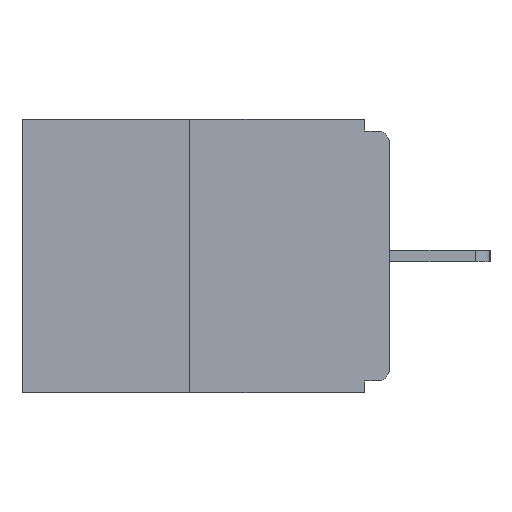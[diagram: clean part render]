
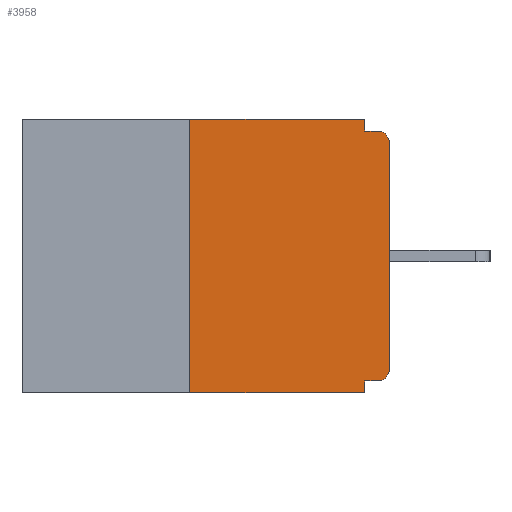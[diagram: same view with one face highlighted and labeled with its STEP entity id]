
A CAD part, left-side view. The second image highlights one B-rep face of the part: STEP entity #3958.
In plain terms, the highlighted planar face has unit normal (-1, 0, 0).
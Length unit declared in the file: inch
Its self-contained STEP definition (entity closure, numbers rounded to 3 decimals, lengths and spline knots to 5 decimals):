
#19 = EDGE_CURVE ( 'NONE', #7502, #7305, #4970, .T. ) ;
#235 = CARTESIAN_POINT ( 'NONE',  ( 0., 0., -0.03 ) ) ;
#389 = EDGE_CURVE ( 'NONE', #7502, #875, #12961, .T. ) ;
#441 = DIRECTION ( 'NONE',  ( 0., 0., -1. ) ) ;
#442 = CARTESIAN_POINT ( 'NONE',  ( 0., 0.015, -0.313 ) ) ;
#732 = CARTESIAN_POINT ( 'NONE',  ( 0., 0.46, 0. ) ) ;
#761 = EDGE_CURVE ( 'NONE', #3249, #5169, #13005, .T. ) ;
#875 = VERTEX_POINT ( 'NONE', #3656 ) ;
#941 = EDGE_CURVE ( 'NONE', #13133, #3249, #1880, .T. ) ;
#1338 = ORIENTED_EDGE ( 'NONE', *, *, #13083, .T. ) ;
#1487 = VERTEX_POINT ( 'NONE', #6552 ) ;
#1519 = ORIENTED_EDGE ( 'NONE', *, *, #2420, .F. ) ;
#1688 = CARTESIAN_POINT ( 'NONE',  ( 0., 0.25, 0. ) ) ;
#1772 = VECTOR ( 'NONE', #441, 39.37008 ) ;
#1880 = LINE ( 'NONE', #3919, #3527 ) ;
#2292 = DIRECTION ( 'NONE',  ( 0., 0., -1. ) ) ;
#2420 = EDGE_CURVE ( 'NONE', #1487, #7305, #12687, .T. ) ;
#2492 = CARTESIAN_POINT ( 'NONE',  ( 0., 0.015, -0.328 ) ) ;
#2587 = VECTOR ( 'NONE', #12234, 39.37008 ) ;
#2642 = DIRECTION ( 'NONE',  ( 0., 0., 1. ) ) ;
#3004 = LINE ( 'NONE', #732, #5067 ) ;
#3183 = ORIENTED_EDGE ( 'NONE', *, *, #941, .T. ) ;
#3249 = VERTEX_POINT ( 'NONE', #235 ) ;
#3290 = EDGE_CURVE ( 'NONE', #8926, #5169, #8013, .T. ) ;
#3332 = FACE_OUTER_BOUND ( 'NONE', #3645, .T. ) ;
#3527 = VECTOR ( 'NONE', #11042, 39.37008 ) ;
#3569 = ORIENTED_EDGE ( 'NONE', *, *, #761, .T. ) ;
#3593 = DIRECTION ( 'NONE',  ( -1., 0., 0. ) ) ;
#3627 = CIRCLE ( 'NONE', #4072, 0.015 ) ;
#3645 = EDGE_LOOP ( 'NONE', ( #9877, #9420, #11605, #1519, #5385, #1338, #3183, #3569, #13025, #5438 ) ) ;
#3656 = CARTESIAN_POINT ( 'NONE',  ( 0., 0.25, 0. ) ) ;
#3919 = CARTESIAN_POINT ( 'NONE',  ( 0., 0., 0. ) ) ;
#3958 = ADVANCED_FACE ( 'NONE', ( #3332 ), #6595, .F. ) ;
#4072 = AXIS2_PLACEMENT_3D ( 'NONE', #442, #11601, #2292 ) ;
#4109 = VERTEX_POINT ( 'NONE', #2492 ) ;
#4481 = LINE ( 'NONE', #8764, #5541 ) ;
#4782 = VECTOR ( 'NONE', #2642, 39.37008 ) ;
#4970 = LINE ( 'NONE', #7951, #2587 ) ;
#5067 = VECTOR ( 'NONE', #8011, 39.37008 ) ;
#5169 = VERTEX_POINT ( 'NONE', #7150 ) ;
#5385 = ORIENTED_EDGE ( 'NONE', *, *, #11361, .F. ) ;
#5438 = ORIENTED_EDGE ( 'NONE', *, *, #5551, .F. ) ;
#5541 = VECTOR ( 'NONE', #10786, 39.37008 ) ;
#5544 = DIRECTION ( 'NONE',  ( 0., -1., 0. ) ) ;
#5551 = EDGE_CURVE ( 'NONE', #6973, #8926, #13355, .T. ) ;
#6093 = CARTESIAN_POINT ( 'NONE',  ( 0., 0.031, 0. ) ) ;
#6552 = CARTESIAN_POINT ( 'NONE',  ( 0., 0.031, -0.328 ) ) ;
#6595 = PLANE ( 'NONE',  #12209 ) ;
#6823 = CARTESIAN_POINT ( 'NONE',  ( 0., 0.031, -0.343 ) ) ;
#6973 = VERTEX_POINT ( 'NONE', #6093 ) ;
#7150 = CARTESIAN_POINT ( 'NONE',  ( 0., 0.015, -0.015 ) ) ;
#7305 = VERTEX_POINT ( 'NONE', #6823 ) ;
#7337 = DIRECTION ( 'NONE',  ( 1., 0., 0. ) ) ;
#7502 = VERTEX_POINT ( 'NONE', #9065 ) ;
#7579 = CARTESIAN_POINT ( 'NONE',  ( 0., 0., -0.015 ) ) ;
#7728 = DIRECTION ( 'NONE',  ( 0., 0., -1. ) ) ;
#7784 = EDGE_CURVE ( 'NONE', #875, #6973, #3004, .T. ) ;
#7874 = CARTESIAN_POINT ( 'NONE',  ( 0., 0.031, -0.015 ) ) ;
#7951 = CARTESIAN_POINT ( 'NONE',  ( 0., 0.46, -0.343 ) ) ;
#8011 = DIRECTION ( 'NONE',  ( 0., -1., 0. ) ) ;
#8013 = LINE ( 'NONE', #7579, #9453 ) ;
#8345 = DIRECTION ( 'NONE',  ( 0., 0., -1. ) ) ;
#8764 = CARTESIAN_POINT ( 'NONE',  ( 0., 0., -0.328 ) ) ;
#8926 = VERTEX_POINT ( 'NONE', #7874 ) ;
#9065 = CARTESIAN_POINT ( 'NONE',  ( 0., 0.25, -0.343 ) ) ;
#9420 = ORIENTED_EDGE ( 'NONE', *, *, #389, .F. ) ;
#9436 = DIRECTION ( 'NONE',  ( 0., 0., -1. ) ) ;
#9453 = VECTOR ( 'NONE', #5544, 39.37008 ) ;
#9562 = CARTESIAN_POINT ( 'NONE',  ( 0., 0.46, 0. ) ) ;
#9806 = CARTESIAN_POINT ( 'NONE',  ( 0., 0.031, -0.343 ) ) ;
#9877 = ORIENTED_EDGE ( 'NONE', *, *, #7784, .F. ) ;
#10300 = CARTESIAN_POINT ( 'NONE',  ( 0., 0.031, 0. ) ) ;
#10714 = CARTESIAN_POINT ( 'NONE',  ( 0., 0.015, -0.03 ) ) ;
#10786 = DIRECTION ( 'NONE',  ( 0., 1., 0. ) ) ;
#10843 = AXIS2_PLACEMENT_3D ( 'NONE', #10714, #3593, #7728 ) ;
#11042 = DIRECTION ( 'NONE',  ( 0., 0., 1. ) ) ;
#11343 = VECTOR ( 'NONE', #8345, 39.37008 ) ;
#11361 = EDGE_CURVE ( 'NONE', #4109, #1487, #4481, .T. ) ;
#11601 = DIRECTION ( 'NONE',  ( -1., 0., 0. ) ) ;
#11605 = ORIENTED_EDGE ( 'NONE', *, *, #19, .T. ) ;
#12209 = AXIS2_PLACEMENT_3D ( 'NONE', #9562, #7337, #9436 ) ;
#12234 = DIRECTION ( 'NONE',  ( 0., -1., 0. ) ) ;
#12687 = LINE ( 'NONE', #9806, #1772 ) ;
#12749 = CARTESIAN_POINT ( 'NONE',  ( 0., 0., -0.313 ) ) ;
#12961 = LINE ( 'NONE', #1688, #4782 ) ;
#13005 = CIRCLE ( 'NONE', #10843, 0.015 ) ;
#13025 = ORIENTED_EDGE ( 'NONE', *, *, #3290, .F. ) ;
#13083 = EDGE_CURVE ( 'NONE', #4109, #13133, #3627, .T. ) ;
#13133 = VERTEX_POINT ( 'NONE', #12749 ) ;
#13355 = LINE ( 'NONE', #10300, #11343 ) ;
